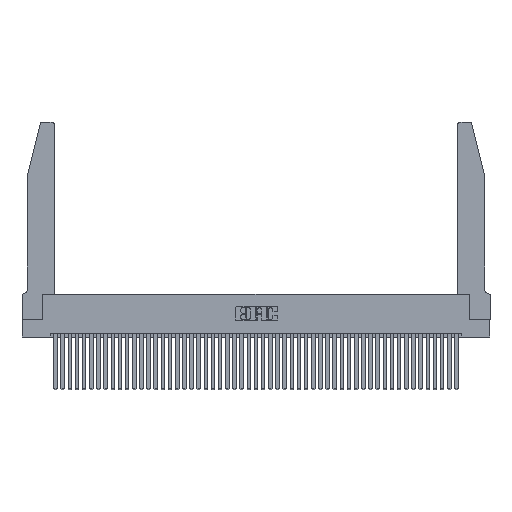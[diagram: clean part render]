
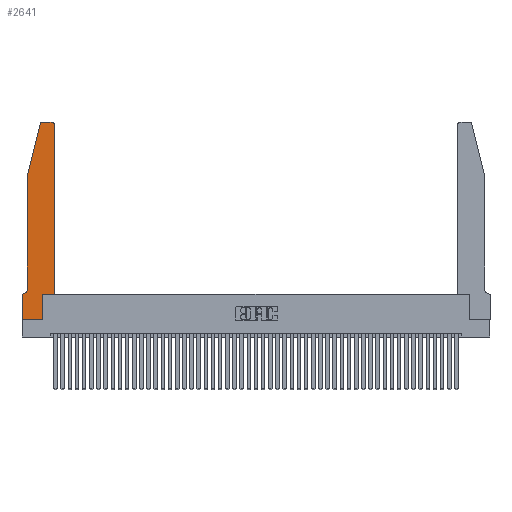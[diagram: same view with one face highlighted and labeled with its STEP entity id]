
A CAD part, top view. The second image highlights one B-rep face of the part: STEP entity #2641.
In plain terms, the highlighted planar face has unit normal (0, 0, 1).
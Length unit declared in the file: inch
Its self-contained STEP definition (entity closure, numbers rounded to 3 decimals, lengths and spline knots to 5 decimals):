
#306 = AXIS2_PLACEMENT_3D ( 'NONE', #490, #26151, #4200 ) ;
#490 = CARTESIAN_POINT ( 'NONE',  ( 0.0055, 0.42, 0.37 ) ) ;
#2103 = AXIS2_PLACEMENT_3D ( 'NONE', #5537, #12974, #38421 ) ;
#2641 = ADVANCED_FACE ( 'NONE', ( #14595 ), #34780, .T. ) ;
#3083 = VERTEX_POINT ( 'NONE', #11662 ) ;
#3187 = VECTOR ( 'NONE', #44833, 39.37008 ) ;
#3666 = CARTESIAN_POINT ( 'NONE',  ( 0., 0.35, 0.37 ) ) ;
#4200 = DIRECTION ( 'NONE',  ( -1., 0., 0. ) ) ;
#4725 = CARTESIAN_POINT ( 'NONE',  ( 0.4205, 2.72, 0.37 ) ) ;
#5482 = VERTEX_POINT ( 'NONE', #34636 ) ;
#5537 = CARTESIAN_POINT ( 'NONE',  ( 0., 0.35, 0.37 ) ) ;
#5668 = EDGE_CURVE ( 'NONE', #17281, #29518, #9019, .T. ) ;
#5854 = CARTESIAN_POINT ( 'NONE',  ( 0.25487, 2.72718, 0.37 ) ) ;
#6163 = VECTOR ( 'NONE', #19286, 39.37008 ) ;
#6219 = LINE ( 'NONE', #13772, #14898 ) ;
#6844 = ORIENTED_EDGE ( 'NONE', *, *, #5668, .T. ) ;
#7406 = VERTEX_POINT ( 'NONE', #5854 ) ;
#8337 = EDGE_CURVE ( 'NONE', #29518, #13358, #43501, .T. ) ;
#8429 = DIRECTION ( 'NONE',  ( 1., 0., 0. ) ) ;
#8926 = EDGE_CURVE ( 'NONE', #5482, #9692, #9371, .T. ) ;
#9019 = LINE ( 'NONE', #36362, #17629 ) ;
#9330 = VERTEX_POINT ( 'NONE', #22486 ) ;
#9371 = LINE ( 'NONE', #16801, #27653 ) ;
#9435 = CIRCLE ( 'NONE', #15115, 0.03 ) ;
#9692 = VERTEX_POINT ( 'NONE', #13542 ) ;
#11445 = CARTESIAN_POINT ( 'NONE',  ( 0.0755, 2., 0.37 ) ) ;
#11662 = CARTESIAN_POINT ( 'NONE',  ( 0.2865, 0.35, 0.37 ) ) ;
#12298 = VECTOR ( 'NONE', #36907, 39.37008 ) ;
#12974 = DIRECTION ( 'NONE',  ( 0., 0., 1. ) ) ;
#13121 = DIRECTION ( 'NONE',  ( -1., 0., 0. ) ) ;
#13358 = VERTEX_POINT ( 'NONE', #31036 ) ;
#13542 = CARTESIAN_POINT ( 'NONE',  ( 0.284, 2.75, 0.37 ) ) ;
#13772 = CARTESIAN_POINT ( 'NONE',  ( 0.4505, 0.35, 0.37 ) ) ;
#14595 = FACE_OUTER_BOUND ( 'NONE', #27723, .T. ) ;
#14898 = VECTOR ( 'NONE', #35576, 39.37008 ) ;
#15032 = CARTESIAN_POINT ( 'NONE',  ( 0.0755, 0.42, 0.37 ) ) ;
#15115 = AXIS2_PLACEMENT_3D ( 'NONE', #19369, #44799, #23049 ) ;
#15127 = ORIENTED_EDGE ( 'NONE', *, *, #44655, .T. ) ;
#15980 = LINE ( 'NONE', #36963, #6163 ) ;
#16801 = CARTESIAN_POINT ( 'NONE',  ( 0.2605, 2.75, 0.37 ) ) ;
#17281 = VERTEX_POINT ( 'NONE', #33781 ) ;
#17629 = VECTOR ( 'NONE', #25545, 39.37008 ) ;
#18009 = EDGE_CURVE ( 'NONE', #9692, #7406, #9435, .T. ) ;
#19286 = DIRECTION ( 'NONE',  ( -0.239, -0.971, 0. ) ) ;
#19369 = CARTESIAN_POINT ( 'NONE',  ( 0.284, 2.72, 0.37 ) ) ;
#21412 = EDGE_CURVE ( 'NONE', #7406, #42997, #15980, .T. ) ;
#22027 = AXIS2_PLACEMENT_3D ( 'NONE', #4725, #30332, #8429 ) ;
#22486 = CARTESIAN_POINT ( 'NONE',  ( 0.4505, 0.35, 0.37 ) ) ;
#22517 = ORIENTED_EDGE ( 'NONE', *, *, #18009, .T. ) ;
#22518 = VECTOR ( 'NONE', #31963, 39.37008 ) ;
#23049 = DIRECTION ( 'NONE',  ( 1., 0., 0. ) ) ;
#23081 = CARTESIAN_POINT ( 'NONE',  ( 0.2865, 0.35, 0.37 ) ) ;
#23330 = VERTEX_POINT ( 'NONE', #15032 ) ;
#23580 = CIRCLE ( 'NONE', #306, 0.07 ) ;
#23630 = ORIENTED_EDGE ( 'NONE', *, *, #35778, .T. ) ;
#23675 = LINE ( 'NONE', #42727, #22518 ) ;
#25545 = DIRECTION ( 'NONE',  ( -1., 0., 0. ) ) ;
#26151 = DIRECTION ( 'NONE',  ( 0., 0., -1. ) ) ;
#26316 = EDGE_CURVE ( 'NONE', #9330, #27982, #35363, .T. ) ;
#27653 = VECTOR ( 'NONE', #13121, 39.37008 ) ;
#27723 = EDGE_LOOP ( 'NONE', ( #35836, #22517, #39999, #33435, #31496, #6844, #35489, #23630, #32348, #37326, #39903, #15127 ) ) ;
#27982 = VERTEX_POINT ( 'NONE', #32822 ) ;
#29518 = VERTEX_POINT ( 'NONE', #3666 ) ;
#30332 = DIRECTION ( 'NONE',  ( 0., 0., 1. ) ) ;
#30526 = LINE ( 'NONE', #11445, #12298 ) ;
#31036 = CARTESIAN_POINT ( 'NONE',  ( 0., 0., 0.37 ) ) ;
#31480 = EDGE_CURVE ( 'NONE', #42997, #23330, #30526, .T. ) ;
#31496 = ORIENTED_EDGE ( 'NONE', *, *, #36680, .T. ) ;
#31645 = CARTESIAN_POINT ( 'NONE',  ( 0.4505, 0.35, 0.37 ) ) ;
#31963 = DIRECTION ( 'NONE',  ( 1., 0., 0. ) ) ;
#32348 = ORIENTED_EDGE ( 'NONE', *, *, #39659, .T. ) ;
#32822 = CARTESIAN_POINT ( 'NONE',  ( 0.4505, 2.72, 0.37 ) ) ;
#33108 = VECTOR ( 'NONE', #42573, 39.37008 ) ;
#33435 = ORIENTED_EDGE ( 'NONE', *, *, #31480, .T. ) ;
#33781 = CARTESIAN_POINT ( 'NONE',  ( 0.0055, 0.35, 0.37 ) ) ;
#34636 = CARTESIAN_POINT ( 'NONE',  ( 0.4205, 2.75, 0.37 ) ) ;
#34780 = PLANE ( 'NONE',  #2103 ) ;
#35363 = LINE ( 'NONE', #31645, #33108 ) ;
#35489 = ORIENTED_EDGE ( 'NONE', *, *, #8337, .T. ) ;
#35576 = DIRECTION ( 'NONE',  ( 1., 0., 0. ) ) ;
#35758 = DIRECTION ( 'NONE',  ( 0., -1., 0. ) ) ;
#35778 = EDGE_CURVE ( 'NONE', #13358, #41633, #23675, .T. ) ;
#35836 = ORIENTED_EDGE ( 'NONE', *, *, #8926, .T. ) ;
#36253 = CARTESIAN_POINT ( 'NONE',  ( 0.0755, 2., 0.37 ) ) ;
#36362 = CARTESIAN_POINT ( 'NONE',  ( 0.0755, 0.35, 0.37 ) ) ;
#36680 = EDGE_CURVE ( 'NONE', #23330, #17281, #23580, .T. ) ;
#36907 = DIRECTION ( 'NONE',  ( 0., -1., 0. ) ) ;
#36963 = CARTESIAN_POINT ( 'NONE',  ( 0.0755, 2., 0.37 ) ) ;
#37326 = ORIENTED_EDGE ( 'NONE', *, *, #43558, .T. ) ;
#38421 = DIRECTION ( 'NONE',  ( 1., 0., 0. ) ) ;
#39659 = EDGE_CURVE ( 'NONE', #41633, #3083, #42030, .T. ) ;
#39903 = ORIENTED_EDGE ( 'NONE', *, *, #26316, .T. ) ;
#39999 = ORIENTED_EDGE ( 'NONE', *, *, #21412, .T. ) ;
#41633 = VERTEX_POINT ( 'NONE', #45867 ) ;
#42030 = LINE ( 'NONE', #23081, #3187 ) ;
#42381 = VECTOR ( 'NONE', #35758, 39.37008 ) ;
#42573 = DIRECTION ( 'NONE',  ( 0., 1., 0. ) ) ;
#42727 = CARTESIAN_POINT ( 'NONE',  ( 0., 0., 0.37 ) ) ;
#42997 = VERTEX_POINT ( 'NONE', #36253 ) ;
#43501 = LINE ( 'NONE', #46536, #42381 ) ;
#43558 = EDGE_CURVE ( 'NONE', #3083, #9330, #6219, .T. ) ;
#44328 = CIRCLE ( 'NONE', #22027, 0.03 ) ;
#44655 = EDGE_CURVE ( 'NONE', #27982, #5482, #44328, .T. ) ;
#44799 = DIRECTION ( 'NONE',  ( 0., 0., 1. ) ) ;
#44833 = DIRECTION ( 'NONE',  ( 0., 1., 0. ) ) ;
#45867 = CARTESIAN_POINT ( 'NONE',  ( 0.2865, 0., 0.37 ) ) ;
#46536 = CARTESIAN_POINT ( 'NONE',  ( 0., 0., 0.37 ) ) ;
